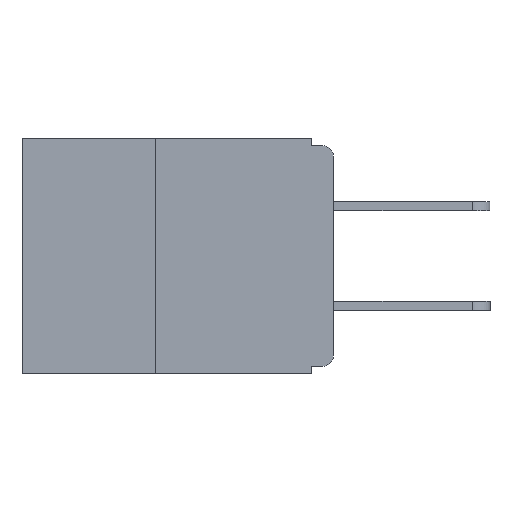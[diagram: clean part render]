
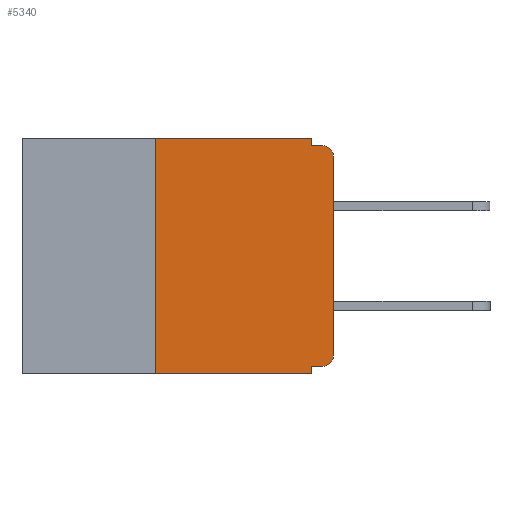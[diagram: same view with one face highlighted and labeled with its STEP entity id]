
A CAD part, left-side view. The second image highlights one B-rep face of the part: STEP entity #5340.
In plain terms, the highlighted planar face has unit normal (-1, 0, 0).
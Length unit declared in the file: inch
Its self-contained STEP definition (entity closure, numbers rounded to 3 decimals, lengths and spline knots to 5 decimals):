
#63 = EDGE_CURVE ( 'NONE', #9134, #3445, #10552, .T. ) ;
#133 = AXIS2_PLACEMENT_3D ( 'NONE', #3827, #411, #11223 ) ;
#411 = DIRECTION ( 'NONE',  ( -1., 0., 0. ) ) ;
#487 = DIRECTION ( 'NONE',  ( 1., 0., 0. ) ) ;
#495 = DIRECTION ( 'NONE',  ( 0., 0., -1. ) ) ;
#617 = LINE ( 'NONE', #8030, #11195 ) ;
#1207 = CARTESIAN_POINT ( 'NONE',  ( 0., 0.031, -0.32 ) ) ;
#1259 = CARTESIAN_POINT ( 'NONE',  ( 0., 0.25, -0.33 ) ) ;
#1274 = EDGE_CURVE ( 'NONE', #7598, #12039, #7134, .T. ) ;
#1478 = ORIENTED_EDGE ( 'NONE', *, *, #63, .F. ) ;
#1543 = DIRECTION ( 'NONE',  ( 0., 0., 1. ) ) ;
#1559 = DIRECTION ( 'NONE',  ( 0., -1., 0. ) ) ;
#1572 = ORIENTED_EDGE ( 'NONE', *, *, #3484, .F. ) ;
#1691 = EDGE_LOOP ( 'NONE', ( #5598, #3979, #9822, #9168, #1572, #1478, #11909, #11055, #9396, #5013 ) ) ;
#1878 = CARTESIAN_POINT ( 'NONE',  ( 0., 0.25, -0.33 ) ) ;
#2108 = LINE ( 'NONE', #10874, #11061 ) ;
#2151 = CARTESIAN_POINT ( 'NONE',  ( 0., 0., -0.025 ) ) ;
#2225 = PLANE ( 'NONE',  #6822 ) ;
#2305 = CARTESIAN_POINT ( 'NONE',  ( 0., 0.015, -0.01 ) ) ;
#2309 = DIRECTION ( 'NONE',  ( 0., 0., -1. ) ) ;
#2413 = DIRECTION ( 'NONE',  ( 0., 1., 0. ) ) ;
#2449 = DIRECTION ( 'NONE',  ( 0., -1., 0. ) ) ;
#2493 = VERTEX_POINT ( 'NONE', #3891 ) ;
#2716 = EDGE_CURVE ( 'NONE', #2493, #10606, #6214, .T. ) ;
#2869 = DIRECTION ( 'NONE',  ( 0., 0., 1. ) ) ;
#3006 = LINE ( 'NONE', #6854, #9013 ) ;
#3010 = EDGE_CURVE ( 'NONE', #9134, #4853, #2108, .T. ) ;
#3383 = CARTESIAN_POINT ( 'NONE',  ( 0., 0., -0.32 ) ) ;
#3417 = LINE ( 'NONE', #9006, #10616 ) ;
#3445 = VERTEX_POINT ( 'NONE', #10830 ) ;
#3484 = EDGE_CURVE ( 'NONE', #3445, #2493, #617, .T. ) ;
#3827 = CARTESIAN_POINT ( 'NONE',  ( 0., 0.015, -0.305 ) ) ;
#3891 = CARTESIAN_POINT ( 'NONE',  ( 0., 0.031, 0. ) ) ;
#3979 = ORIENTED_EDGE ( 'NONE', *, *, #9336, .T. ) ;
#4202 = EDGE_CURVE ( 'NONE', #10606, #4691, #3417, .T. ) ;
#4691 = VERTEX_POINT ( 'NONE', #2305 ) ;
#4853 = VERTEX_POINT ( 'NONE', #10143 ) ;
#5013 = ORIENTED_EDGE ( 'NONE', *, *, #6058, .T. ) ;
#5037 = AXIS2_PLACEMENT_3D ( 'NONE', #10972, #10841, #495 ) ;
#5340 = ADVANCED_FACE ( 'NONE', ( #6003 ), #2225, .F. ) ;
#5598 = ORIENTED_EDGE ( 'NONE', *, *, #1274, .T. ) ;
#6003 = FACE_OUTER_BOUND ( 'NONE', #1691, .T. ) ;
#6016 = DIRECTION ( 'NONE',  ( 0., -1., 0. ) ) ;
#6058 = EDGE_CURVE ( 'NONE', #10644, #7598, #9589, .T. ) ;
#6214 = LINE ( 'NONE', #9662, #12087 ) ;
#6822 = AXIS2_PLACEMENT_3D ( 'NONE', #10717, #487, #2309 ) ;
#6854 = CARTESIAN_POINT ( 'NONE',  ( 0., 0.031, -0.33 ) ) ;
#7134 = LINE ( 'NONE', #10901, #11243 ) ;
#7598 = VERTEX_POINT ( 'NONE', #10737 ) ;
#8030 = CARTESIAN_POINT ( 'NONE',  ( 0., 0.437, 0. ) ) ;
#8183 = CARTESIAN_POINT ( 'NONE',  ( 0., 0.015, -0.32 ) ) ;
#8643 = LINE ( 'NONE', #3383, #11575 ) ;
#8797 = DIRECTION ( 'NONE',  ( 0., 0., -1. ) ) ;
#8821 = EDGE_CURVE ( 'NONE', #10644, #9402, #8643, .T. ) ;
#9006 = CARTESIAN_POINT ( 'NONE',  ( 0., 0., -0.01 ) ) ;
#9013 = VECTOR ( 'NONE', #8797, 39.37008 ) ;
#9098 = CARTESIAN_POINT ( 'NONE',  ( 0., 0.031, -0.01 ) ) ;
#9134 = VERTEX_POINT ( 'NONE', #1259 ) ;
#9168 = ORIENTED_EDGE ( 'NONE', *, *, #2716, .F. ) ;
#9336 = EDGE_CURVE ( 'NONE', #12039, #4691, #12146, .T. ) ;
#9396 = ORIENTED_EDGE ( 'NONE', *, *, #8821, .F. ) ;
#9402 = VERTEX_POINT ( 'NONE', #1207 ) ;
#9589 = CIRCLE ( 'NONE', #133, 0.015 ) ;
#9662 = CARTESIAN_POINT ( 'NONE',  ( 0., 0.031, 0. ) ) ;
#9822 = ORIENTED_EDGE ( 'NONE', *, *, #4202, .F. ) ;
#9857 = DIRECTION ( 'NONE',  ( 0., 0., -1. ) ) ;
#10143 = CARTESIAN_POINT ( 'NONE',  ( 0., 0.031, -0.33 ) ) ;
#10552 = LINE ( 'NONE', #1878, #12151 ) ;
#10606 = VERTEX_POINT ( 'NONE', #9098 ) ;
#10616 = VECTOR ( 'NONE', #2449, 39.37008 ) ;
#10644 = VERTEX_POINT ( 'NONE', #8183 ) ;
#10717 = CARTESIAN_POINT ( 'NONE',  ( 0., 0.437, 0. ) ) ;
#10737 = CARTESIAN_POINT ( 'NONE',  ( 0., 0., -0.305 ) ) ;
#10830 = CARTESIAN_POINT ( 'NONE',  ( 0., 0.25, 0. ) ) ;
#10841 = DIRECTION ( 'NONE',  ( -1., 0., 0. ) ) ;
#10874 = CARTESIAN_POINT ( 'NONE',  ( 0., 0.437, -0.33 ) ) ;
#10901 = CARTESIAN_POINT ( 'NONE',  ( 0., 0., 0. ) ) ;
#10972 = CARTESIAN_POINT ( 'NONE',  ( 0., 0.015, -0.025 ) ) ;
#11055 = ORIENTED_EDGE ( 'NONE', *, *, #11644, .F. ) ;
#11061 = VECTOR ( 'NONE', #1559, 39.37008 ) ;
#11195 = VECTOR ( 'NONE', #6016, 39.37008 ) ;
#11223 = DIRECTION ( 'NONE',  ( 0., 0., -1. ) ) ;
#11243 = VECTOR ( 'NONE', #1543, 39.37008 ) ;
#11575 = VECTOR ( 'NONE', #2413, 39.37008 ) ;
#11644 = EDGE_CURVE ( 'NONE', #9402, #4853, #3006, .T. ) ;
#11909 = ORIENTED_EDGE ( 'NONE', *, *, #3010, .T. ) ;
#12039 = VERTEX_POINT ( 'NONE', #2151 ) ;
#12087 = VECTOR ( 'NONE', #9857, 39.37008 ) ;
#12146 = CIRCLE ( 'NONE', #5037, 0.015 ) ;
#12151 = VECTOR ( 'NONE', #2869, 39.37008 ) ;
